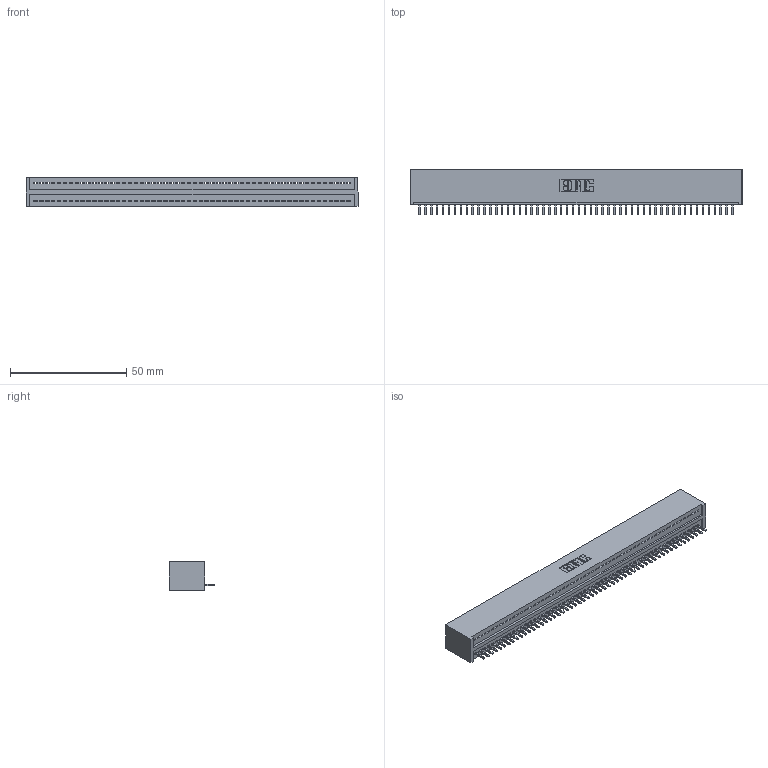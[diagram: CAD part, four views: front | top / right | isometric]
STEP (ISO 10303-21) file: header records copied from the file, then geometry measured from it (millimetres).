
FILE_DESCRIPTION (( 'STEP AP203' ), '1' );
FILE_NAME ('325-054-520-101.STEP', '2020-02-25T00:52:34', ( '' ), ( '' ), 'SwSTEP 2.0', 'SolidWorks 2016', '' );
FILE_SCHEMA (( 'CONFIG_CONTROL_DESIGN' ));
Length unit declared in the file: inch
Products named in the file (3): 325-054-520-101; 325 Part_Lugless; 325-292-001_325-293-120
Assembly tree (55 placements, depth 2):
  325-054-520-101
    325 Part_Lugless
    325-292-001_325-293-120  x54
Bounding box: 142.8 x 19.68 x 12.45 mm (x, y, z)
Volume: 18654.8 mm3; surface area: 20506.5 mm2
Topology: 55 solids, 55 shells, 3238 faces, 9791 edges, 6454 vertices
Faces by surface type: plane 2334, cylinder 904
Entity records: 31201 total; most frequent: CARTESIAN_POINT 5388, ORIENTED_EDGE 5378, DIRECTION 4513, EDGE_CURVE 2689, LINE 2569, VECTOR 2569, VERTEX_POINT 1790, AXIS2_PLACEMENT_3D 972
